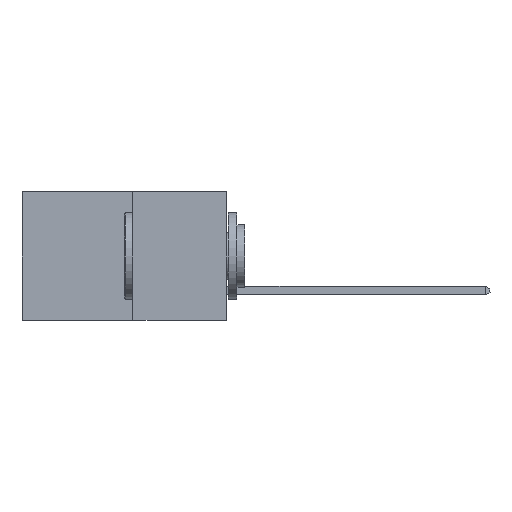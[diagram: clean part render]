
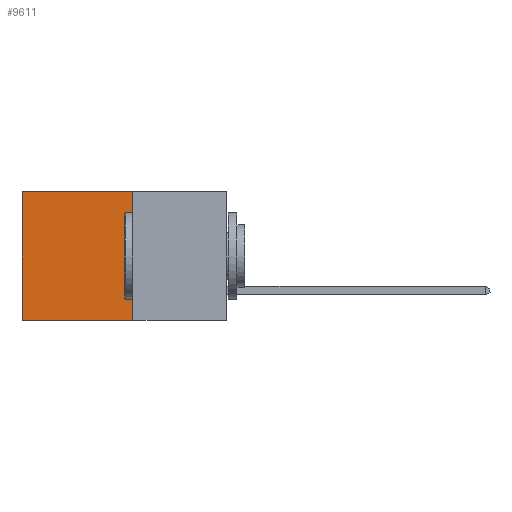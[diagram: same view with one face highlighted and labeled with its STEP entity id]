
A CAD part, left-side view. The second image highlights one B-rep face of the part: STEP entity #9611.
In plain terms, the highlighted planar face has unit normal (-1, 0, 0).
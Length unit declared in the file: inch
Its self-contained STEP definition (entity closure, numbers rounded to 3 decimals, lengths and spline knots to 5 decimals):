
#402 = ORIENTED_EDGE ( 'NONE', *, *, #9806, .T. ) ;
#531 = DIRECTION ( 'NONE',  ( 0., 1., 0. ) ) ;
#547 = CARTESIAN_POINT ( 'NONE',  ( 0.277, 0.27, 0. ) ) ;
#892 = ORIENTED_EDGE ( 'NONE', *, *, #5171, .T. ) ;
#981 = DIRECTION ( 'NONE',  ( 0., 1., 0. ) ) ;
#1451 = VECTOR ( 'NONE', #531, 39.37008 ) ;
#1473 = DIRECTION ( 'NONE',  ( 0., 0., -1. ) ) ;
#1942 = DIRECTION ( 'NONE',  ( 1., 0., 0. ) ) ;
#2071 = CARTESIAN_POINT ( 'NONE',  ( 0.277, 0.27, -0.37 ) ) ;
#2241 = VERTEX_POINT ( 'NONE', #9319 ) ;
#2251 = VERTEX_POINT ( 'NONE', #547 ) ;
#3355 = CARTESIAN_POINT ( 'NONE',  ( 0.277, 0.59, -0.37 ) ) ;
#3603 = LINE ( 'NONE', #2071, #5497 ) ;
#3829 = ORIENTED_EDGE ( 'NONE', *, *, #4299, .F. ) ;
#4299 = EDGE_CURVE ( 'NONE', #2251, #9122, #3603, .T. ) ;
#4428 = CARTESIAN_POINT ( 'NONE',  ( 0.277, 0.27, -0.37 ) ) ;
#4702 = VERTEX_POINT ( 'NONE', #6073 ) ;
#5034 = CARTESIAN_POINT ( 'NONE',  ( 0.277, 0.27, -0.37 ) ) ;
#5171 = EDGE_CURVE ( 'NONE', #2241, #4702, #10293, .T. ) ;
#5497 = VECTOR ( 'NONE', #1473, 39.37008 ) ;
#6073 = CARTESIAN_POINT ( 'NONE',  ( 0.277, 0.59, -0.37 ) ) ;
#6269 = CARTESIAN_POINT ( 'NONE',  ( 0.277, 0.27, 0. ) ) ;
#6775 = CARTESIAN_POINT ( 'NONE',  ( 0.277, 0.27, -0.37 ) ) ;
#7266 = LINE ( 'NONE', #5034, #9132 ) ;
#7499 = EDGE_LOOP ( 'NONE', ( #892, #8515, #3829, #402 ) ) ;
#7579 = DIRECTION ( 'NONE',  ( 0., 0., -1. ) ) ;
#7846 = AXIS2_PLACEMENT_3D ( 'NONE', #6775, #1942, #7579 ) ;
#7884 = LINE ( 'NONE', #6269, #1451 ) ;
#8270 = VECTOR ( 'NONE', #8876, 39.37008 ) ;
#8345 = PLANE ( 'NONE',  #7846 ) ;
#8515 = ORIENTED_EDGE ( 'NONE', *, *, #10288, .F. ) ;
#8876 = DIRECTION ( 'NONE',  ( 0., 0., -1. ) ) ;
#9122 = VERTEX_POINT ( 'NONE', #4428 ) ;
#9132 = VECTOR ( 'NONE', #981, 39.37008 ) ;
#9319 = CARTESIAN_POINT ( 'NONE',  ( 0.277, 0.59, 0. ) ) ;
#9611 = ADVANCED_FACE ( 'NONE', ( #9726 ), #8345, .F. ) ;
#9726 = FACE_OUTER_BOUND ( 'NONE', #7499, .T. ) ;
#9806 = EDGE_CURVE ( 'NONE', #2251, #2241, #7884, .T. ) ;
#10288 = EDGE_CURVE ( 'NONE', #9122, #4702, #7266, .T. ) ;
#10293 = LINE ( 'NONE', #3355, #8270 ) ;
